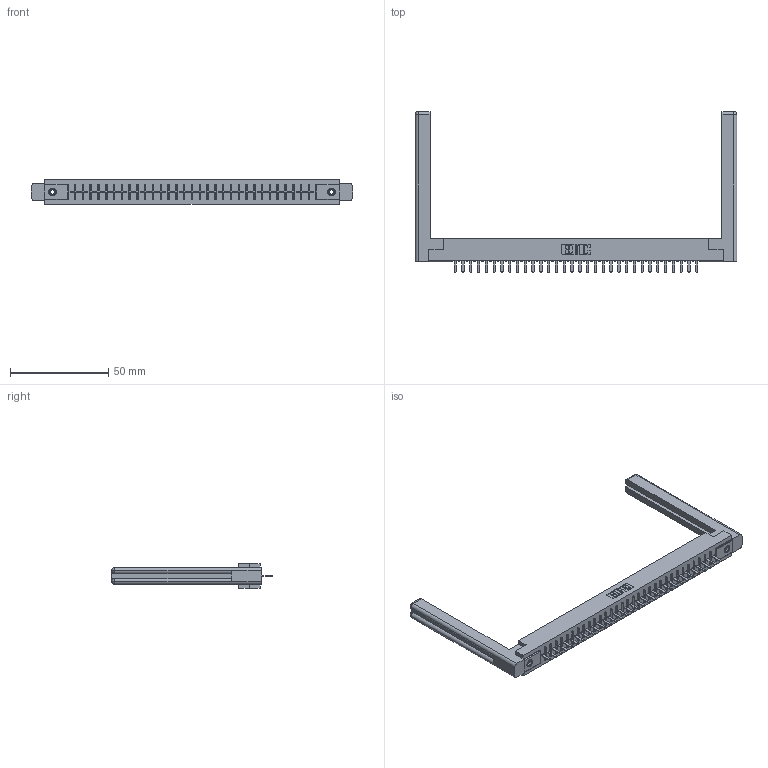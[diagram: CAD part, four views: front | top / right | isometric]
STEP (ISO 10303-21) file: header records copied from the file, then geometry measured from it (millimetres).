
FILE_DESCRIPTION (( 'STEP AP203' ), '1' );
FILE_NAME ('316-032-520-158.STEP', '2018-07-31T03:42:15', ( '' ), ( '' ), 'SwSTEP 2.0', 'SolidWorks 2016', '' );
FILE_SCHEMA (( 'CONFIG_CONTROL_DESIGN' ));
Length unit declared in the file: inch
Products named in the file (5): 306-290-001_120; 345-250-001_345-250-001-102; 307-220-058; 316-032-520-158; 306 Part_.156 Dia
Assembly tree (37 placements, depth 2):
  316-032-520-158
    306 Part_.156 Dia
    306-290-001_120  x32
    345-250-001_345-250-001-102  x2
    307-220-058  x2
Bounding box: 163.42 x 81.76 x 12.7 mm (x, y, z)
Volume: 25063.4 mm3; surface area: 23484.8 mm2
Topology: 37 solids, 37 shells, 2498 faces, 6974 edges, 4464 vertices
Faces by surface type: plane 1656, cylinder 690, sphere 128, cone 12, torus 12
Entity records: 33726 total; most frequent: CARTESIAN_POINT 5670, ORIENTED_EDGE 5562, DIRECTION 5547, EDGE_CURVE 2781, LINE 2165, VECTOR 2165, VERTEX_POINT 1760, AXIS2_PLACEMENT_3D 1691
